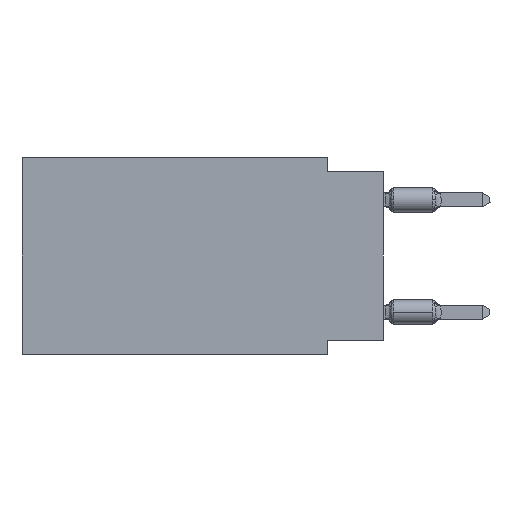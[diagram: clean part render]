
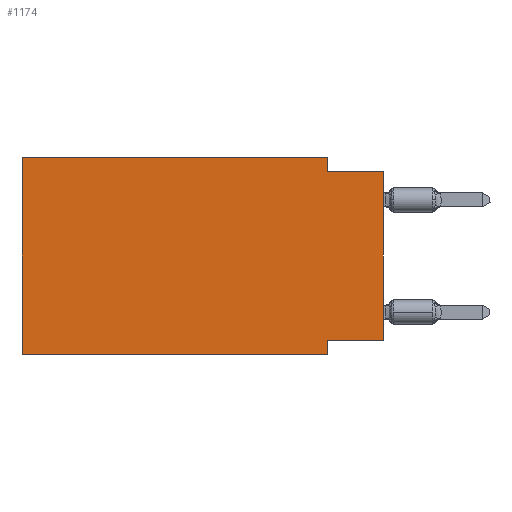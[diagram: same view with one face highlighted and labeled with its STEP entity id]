
A CAD part, left-side view. The second image highlights one B-rep face of the part: STEP entity #1174.
In plain terms, the highlighted planar face has unit normal (-1, 0, 0).
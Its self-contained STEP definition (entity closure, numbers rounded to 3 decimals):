
#15 = CARTESIAN_POINT ( 'NONE',  ( 0., 16.383, -8.89 ) ) ;
#275 = LINE ( 'NONE', #5835, #37484 ) ;
#459 = DIRECTION ( 'NONE',  ( 0., 0., -1. ) ) ;
#954 = AXIS2_PLACEMENT_3D ( 'NONE', #23626, #40454, #33431 ) ;
#1174 = ADVANCED_FACE ( 'NONE', ( #20659 ), #14727, .F. ) ;
#1310 = CARTESIAN_POINT ( 'NONE',  ( 0., 0., -8.255 ) ) ;
#2737 = ORIENTED_EDGE ( 'NONE', *, *, #40577, .F. ) ;
#3219 = CARTESIAN_POINT ( 'NONE',  ( 0., 0., -0.635 ) ) ;
#3260 = LINE ( 'NONE', #23000, #41906 ) ;
#5835 = CARTESIAN_POINT ( 'NONE',  ( 0., 0., -8.255 ) ) ;
#5957 = ORIENTED_EDGE ( 'NONE', *, *, #9067, .F. ) ;
#6662 = LINE ( 'NONE', #27050, #16729 ) ;
#6851 = CARTESIAN_POINT ( 'NONE',  ( 0., 2.54, -8.89 ) ) ;
#7391 = EDGE_CURVE ( 'NONE', #13867, #27116, #12771, .T. ) ;
#7513 = ORIENTED_EDGE ( 'NONE', *, *, #24611, .T. ) ;
#8353 = LINE ( 'NONE', #40475, #25005 ) ;
#8593 = CARTESIAN_POINT ( 'NONE',  ( 0., 0., -0.635 ) ) ;
#9067 = EDGE_CURVE ( 'NONE', #39533, #27116, #23399, .T. ) ;
#9245 = DIRECTION ( 'NONE',  ( 0., 1., 0. ) ) ;
#11561 = ORIENTED_EDGE ( 'NONE', *, *, #29426, .F. ) ;
#12771 = LINE ( 'NONE', #22102, #13550 ) ;
#12972 = DIRECTION ( 'NONE',  ( 0., -1., 0. ) ) ;
#13049 = VECTOR ( 'NONE', #21549, 1000. ) ;
#13430 = EDGE_CURVE ( 'NONE', #38220, #39533, #275, .T. ) ;
#13550 = VECTOR ( 'NONE', #12972, 1000. ) ;
#13867 = VERTEX_POINT ( 'NONE', #15 ) ;
#14102 = EDGE_LOOP ( 'NONE', ( #7513, #39717, #28011, #11561, #2737, #14645, #5957, #39895 ) ) ;
#14592 = VECTOR ( 'NONE', #19259, 1000. ) ;
#14645 = ORIENTED_EDGE ( 'NONE', *, *, #7391, .T. ) ;
#14727 = PLANE ( 'NONE',  #954 ) ;
#15253 = VERTEX_POINT ( 'NONE', #28939 ) ;
#16729 = VECTOR ( 'NONE', #19617, 1000. ) ;
#19259 = DIRECTION ( 'NONE',  ( 0., 0., -1. ) ) ;
#19617 = DIRECTION ( 'NONE',  ( 0., -1., 0. ) ) ;
#20294 = CARTESIAN_POINT ( 'NONE',  ( 0., 16.383, 0. ) ) ;
#20659 = FACE_OUTER_BOUND ( 'NONE', #14102, .T. ) ;
#21549 = DIRECTION ( 'NONE',  ( 0., -1., 0. ) ) ;
#21780 = VERTEX_POINT ( 'NONE', #20294 ) ;
#22102 = CARTESIAN_POINT ( 'NONE',  ( 0., 16.383, -8.89 ) ) ;
#23000 = CARTESIAN_POINT ( 'NONE',  ( 0., 0., 0. ) ) ;
#23399 = LINE ( 'NONE', #39797, #33343 ) ;
#23626 = CARTESIAN_POINT ( 'NONE',  ( 0., 16.383, 0. ) ) ;
#24304 = LINE ( 'NONE', #8593, #13049 ) ;
#24611 = EDGE_CURVE ( 'NONE', #38220, #35101, #3260, .T. ) ;
#25005 = VECTOR ( 'NONE', #27709, 1000. ) ;
#25431 = LINE ( 'NONE', #32675, #14592 ) ;
#25570 = DIRECTION ( 'NONE',  ( 0., 0., 1. ) ) ;
#27050 = CARTESIAN_POINT ( 'NONE',  ( 0., 16.383, 0. ) ) ;
#27116 = VERTEX_POINT ( 'NONE', #6851 ) ;
#27709 = DIRECTION ( 'NONE',  ( 0., 0., 1. ) ) ;
#28011 = ORIENTED_EDGE ( 'NONE', *, *, #35846, .F. ) ;
#28939 = CARTESIAN_POINT ( 'NONE',  ( 0., 2.54, 0. ) ) ;
#29426 = EDGE_CURVE ( 'NONE', #21780, #15253, #6662, .T. ) ;
#32479 = EDGE_CURVE ( 'NONE', #34710, #35101, #24304, .T. ) ;
#32675 = CARTESIAN_POINT ( 'NONE',  ( 0., 2.54, 0. ) ) ;
#32761 = CARTESIAN_POINT ( 'NONE',  ( 0., 2.54, -8.255 ) ) ;
#33343 = VECTOR ( 'NONE', #459, 1000. ) ;
#33431 = DIRECTION ( 'NONE',  ( 0., 0., -1. ) ) ;
#34710 = VERTEX_POINT ( 'NONE', #35637 ) ;
#35101 = VERTEX_POINT ( 'NONE', #3219 ) ;
#35637 = CARTESIAN_POINT ( 'NONE',  ( 0., 2.54, -0.635 ) ) ;
#35846 = EDGE_CURVE ( 'NONE', #15253, #34710, #25431, .T. ) ;
#37484 = VECTOR ( 'NONE', #9245, 1000. ) ;
#38220 = VERTEX_POINT ( 'NONE', #1310 ) ;
#39533 = VERTEX_POINT ( 'NONE', #32761 ) ;
#39717 = ORIENTED_EDGE ( 'NONE', *, *, #32479, .F. ) ;
#39797 = CARTESIAN_POINT ( 'NONE',  ( 0., 2.54, -8.89 ) ) ;
#39895 = ORIENTED_EDGE ( 'NONE', *, *, #13430, .F. ) ;
#40454 = DIRECTION ( 'NONE',  ( 1., 0., 0. ) ) ;
#40475 = CARTESIAN_POINT ( 'NONE',  ( 0., 16.383, 0. ) ) ;
#40577 = EDGE_CURVE ( 'NONE', #13867, #21780, #8353, .T. ) ;
#41906 = VECTOR ( 'NONE', #25570, 1000. ) ;
